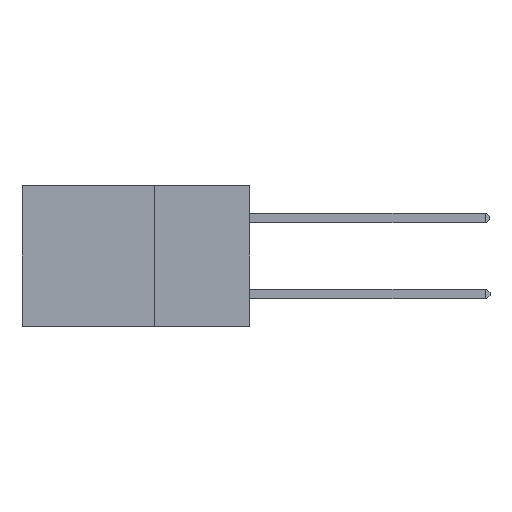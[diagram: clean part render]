
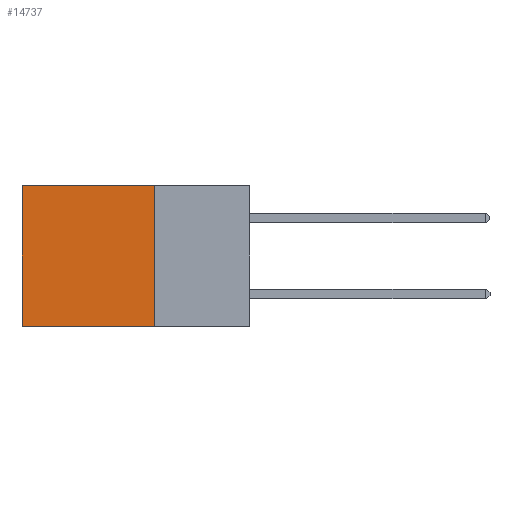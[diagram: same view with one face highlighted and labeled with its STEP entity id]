
A CAD part, left-side view. The second image highlights one B-rep face of the part: STEP entity #14737.
In plain terms, the highlighted planar face has unit normal (-1, 0, 0).
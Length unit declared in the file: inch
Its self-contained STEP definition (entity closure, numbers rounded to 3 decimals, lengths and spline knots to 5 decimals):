
#193 = ORIENTED_EDGE ( 'NONE', *, *, #23414, .F. ) ;
#1496 = DIRECTION ( 'NONE',  ( 1., 0., 0. ) ) ;
#2350 = EDGE_CURVE ( 'NONE', #9109, #2747, #4926, .T. ) ;
#2747 = VERTEX_POINT ( 'NONE', #17091 ) ;
#2871 = ORIENTED_EDGE ( 'NONE', *, *, #2350, .T. ) ;
#3256 = EDGE_CURVE ( 'NONE', #16228, #9109, #22290, .T. ) ;
#3559 = CARTESIAN_POINT ( 'NONE',  ( 0.2875, 0.6, 0. ) ) ;
#4217 = FACE_OUTER_BOUND ( 'NONE', #9697, .T. ) ;
#4926 = LINE ( 'NONE', #21260, #10060 ) ;
#5673 = DIRECTION ( 'NONE',  ( 0., 0., -1. ) ) ;
#6826 = VECTOR ( 'NONE', #15068, 39.37008 ) ;
#7824 = CARTESIAN_POINT ( 'NONE',  ( 0.2875, 0.25, -0.37 ) ) ;
#8003 = DIRECTION ( 'NONE',  ( 0., 1., 0. ) ) ;
#8599 = CARTESIAN_POINT ( 'NONE',  ( 0.2875, 0.25, 0. ) ) ;
#9109 = VERTEX_POINT ( 'NONE', #3559 ) ;
#9252 = VECTOR ( 'NONE', #8003, 39.37008 ) ;
#9697 = EDGE_LOOP ( 'NONE', ( #2871, #193, #13965, #15967 ) ) ;
#10060 = VECTOR ( 'NONE', #5673, 39.37008 ) ;
#10224 = AXIS2_PLACEMENT_3D ( 'NONE', #8599, #1496, #13517 ) ;
#10328 = CARTESIAN_POINT ( 'NONE',  ( 0.2875, 0.25, -0.37 ) ) ;
#11509 = CARTESIAN_POINT ( 'NONE',  ( 0.2875, 0.25, 0. ) ) ;
#12342 = PLANE ( 'NONE',  #10224 ) ;
#13292 = VECTOR ( 'NONE', #18066, 39.37008 ) ;
#13517 = DIRECTION ( 'NONE',  ( 0., 0., -1. ) ) ;
#13965 = ORIENTED_EDGE ( 'NONE', *, *, #15525, .F. ) ;
#14392 = LINE ( 'NONE', #7824, #9252 ) ;
#14737 = ADVANCED_FACE ( 'NONE', ( #4217 ), #12342, .F. ) ;
#15068 = DIRECTION ( 'NONE',  ( 0., 1., 0. ) ) ;
#15525 = EDGE_CURVE ( 'NONE', #16228, #23043, #18425, .T. ) ;
#15833 = CARTESIAN_POINT ( 'NONE',  ( 0.2875, 0.25, 0. ) ) ;
#15967 = ORIENTED_EDGE ( 'NONE', *, *, #3256, .T. ) ;
#16228 = VERTEX_POINT ( 'NONE', #15833 ) ;
#17091 = CARTESIAN_POINT ( 'NONE',  ( 0.2875, 0.6, -0.37 ) ) ;
#18066 = DIRECTION ( 'NONE',  ( 0., 0., -1. ) ) ;
#18149 = CARTESIAN_POINT ( 'NONE',  ( 0.2875, 0.25, 0. ) ) ;
#18425 = LINE ( 'NONE', #18149, #13292 ) ;
#21260 = CARTESIAN_POINT ( 'NONE',  ( 0.2875, 0.6, 0. ) ) ;
#22290 = LINE ( 'NONE', #11509, #6826 ) ;
#23043 = VERTEX_POINT ( 'NONE', #10328 ) ;
#23414 = EDGE_CURVE ( 'NONE', #23043, #2747, #14392, .T. ) ;
